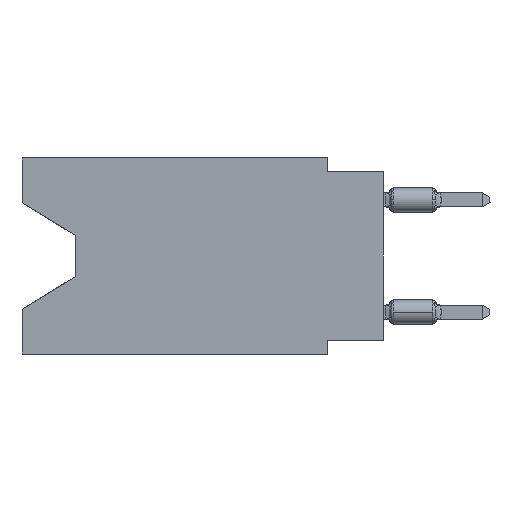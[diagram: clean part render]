
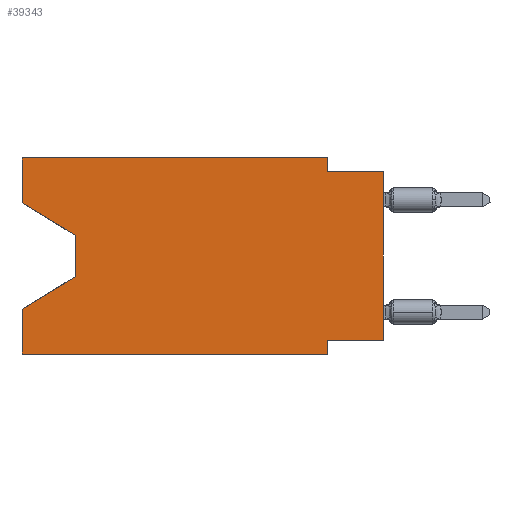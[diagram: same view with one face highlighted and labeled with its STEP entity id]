
A CAD part, left-side view. The second image highlights one B-rep face of the part: STEP entity #39343.
In plain terms, the highlighted planar face has unit normal (-1, 0, 0).
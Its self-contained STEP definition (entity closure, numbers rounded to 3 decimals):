
#518 = DIRECTION ( 'NONE',  ( 0., -1., 0. ) ) ;
#731 = DIRECTION ( 'NONE',  ( 0., -1., 0. ) ) ;
#1422 = CARTESIAN_POINT ( 'NONE',  ( 0., 13.97, -3.505 ) ) ;
#1849 = VERTEX_POINT ( 'NONE', #2627 ) ;
#1996 = VECTOR ( 'NONE', #51085, 1000. ) ;
#2087 = EDGE_LOOP ( 'NONE', ( #16114, #37266, #36667, #16920, #6599, #61075, #36637, #40089, #30793, #2458, #24919, #53079 ) ) ;
#2458 = ORIENTED_EDGE ( 'NONE', *, *, #10654, .F. ) ;
#2627 = CARTESIAN_POINT ( 'NONE',  ( 0., 2.54, -8.255 ) ) ;
#3861 = CARTESIAN_POINT ( 'NONE',  ( 0., 16.383, -8.89 ) ) ;
#4676 = CARTESIAN_POINT ( 'NONE',  ( 0., 0., -0.635 ) ) ;
#5879 = LINE ( 'NONE', #40136, #1996 ) ;
#6353 = CARTESIAN_POINT ( 'NONE',  ( 0., 16.383, -8.89 ) ) ;
#6599 = ORIENTED_EDGE ( 'NONE', *, *, #56846, .T. ) ;
#6923 = CARTESIAN_POINT ( 'NONE',  ( 0., 16.383, 0. ) ) ;
#7086 = LINE ( 'NONE', #69049, #21964 ) ;
#8711 = LINE ( 'NONE', #36781, #38180 ) ;
#8749 = DIRECTION ( 'NONE',  ( 0., 0., -1. ) ) ;
#9603 = CARTESIAN_POINT ( 'NONE',  ( 0., 16.383, -2.038 ) ) ;
#10057 = DIRECTION ( 'NONE',  ( 0., 0., -1. ) ) ;
#10330 = DIRECTION ( 'NONE',  ( 0., 0., 1. ) ) ;
#10654 = EDGE_CURVE ( 'NONE', #14578, #63282, #7086, .T. ) ;
#12421 = VECTOR ( 'NONE', #10057, 1000. ) ;
#12551 = EDGE_CURVE ( 'NONE', #14363, #37885, #18939, .T. ) ;
#12868 = VERTEX_POINT ( 'NONE', #9603 ) ;
#13002 = CARTESIAN_POINT ( 'NONE',  ( 0., 16.383, 0. ) ) ;
#14363 = VERTEX_POINT ( 'NONE', #3861 ) ;
#14437 = VECTOR ( 'NONE', #518, 1000. ) ;
#14578 = VERTEX_POINT ( 'NONE', #28635 ) ;
#14747 = LINE ( 'NONE', #59226, #44307 ) ;
#15629 = VECTOR ( 'NONE', #36415, 1000. ) ;
#16114 = ORIENTED_EDGE ( 'NONE', *, *, #65312, .T. ) ;
#16920 = ORIENTED_EDGE ( 'NONE', *, *, #12551, .F. ) ;
#17519 = LINE ( 'NONE', #56531, #51756 ) ;
#17659 = VECTOR ( 'NONE', #30242, 1000. ) ;
#18939 = LINE ( 'NONE', #57948, #17659 ) ;
#19526 = VERTEX_POINT ( 'NONE', #44234 ) ;
#20314 = CARTESIAN_POINT ( 'NONE',  ( 0., 13.97, -5.385 ) ) ;
#21296 = EDGE_CURVE ( 'NONE', #25168, #22337, #37775, .T. ) ;
#21964 = VECTOR ( 'NONE', #52293, 1000. ) ;
#22337 = VERTEX_POINT ( 'NONE', #20314 ) ;
#24919 = ORIENTED_EDGE ( 'NONE', *, *, #62285, .F. ) ;
#25168 = VERTEX_POINT ( 'NONE', #1422 ) ;
#26548 = EDGE_CURVE ( 'NONE', #22337, #37885, #8711, .T. ) ;
#27928 = CARTESIAN_POINT ( 'NONE',  ( 0., 2.54, -0.635 ) ) ;
#28635 = CARTESIAN_POINT ( 'NONE',  ( 0., 2.54, 0. ) ) ;
#29159 = DIRECTION ( 'NONE',  ( 0., 0., -1. ) ) ;
#29641 = VERTEX_POINT ( 'NONE', #70149 ) ;
#30242 = DIRECTION ( 'NONE',  ( 0., 0., 1. ) ) ;
#30793 = ORIENTED_EDGE ( 'NONE', *, *, #40383, .F. ) ;
#31771 = VECTOR ( 'NONE', #10330, 1000. ) ;
#31847 = CARTESIAN_POINT ( 'NONE',  ( 0., 0., 0. ) ) ;
#35004 = EDGE_CURVE ( 'NONE', #19526, #1849, #5879, .T. ) ;
#35238 = VECTOR ( 'NONE', #47574, 1000. ) ;
#35347 = LINE ( 'NONE', #45940, #15629 ) ;
#36104 = CARTESIAN_POINT ( 'NONE',  ( 0., 2.54, -8.89 ) ) ;
#36415 = DIRECTION ( 'NONE',  ( 0., 0., 1. ) ) ;
#36637 = ORIENTED_EDGE ( 'NONE', *, *, #35004, .F. ) ;
#36667 = ORIENTED_EDGE ( 'NONE', *, *, #26548, .T. ) ;
#36781 = CARTESIAN_POINT ( 'NONE',  ( 0., 13.97, -5.385 ) ) ;
#37266 = ORIENTED_EDGE ( 'NONE', *, *, #21296, .T. ) ;
#37775 = LINE ( 'NONE', #60020, #12421 ) ;
#37885 = VERTEX_POINT ( 'NONE', #42711 ) ;
#38180 = VECTOR ( 'NONE', #47729, 1000. ) ;
#39218 = EDGE_CURVE ( 'NONE', #19526, #62628, #59557, .T. ) ;
#39343 = ADVANCED_FACE ( 'NONE', ( #55182 ), #56879, .F. ) ;
#40089 = ORIENTED_EDGE ( 'NONE', *, *, #39218, .T. ) ;
#40136 = CARTESIAN_POINT ( 'NONE',  ( 0., 0., -8.255 ) ) ;
#40383 = EDGE_CURVE ( 'NONE', #63282, #62628, #14747, .T. ) ;
#42711 = CARTESIAN_POINT ( 'NONE',  ( 0., 16.383, -6.852 ) ) ;
#44234 = CARTESIAN_POINT ( 'NONE',  ( 0., 0., -8.255 ) ) ;
#44307 = VECTOR ( 'NONE', #58488, 1000. ) ;
#45940 = CARTESIAN_POINT ( 'NONE',  ( 0., 16.383, 0. ) ) ;
#46505 = CARTESIAN_POINT ( 'NONE',  ( 0., 16.383, -2.038 ) ) ;
#47228 = LINE ( 'NONE', #46505, #35238 ) ;
#47574 = DIRECTION ( 'NONE',  ( 0., -0.855, -0.519 ) ) ;
#47729 = DIRECTION ( 'NONE',  ( 0., 0.855, -0.519 ) ) ;
#51085 = DIRECTION ( 'NONE',  ( 0., 1., 0. ) ) ;
#51756 = VECTOR ( 'NONE', #731, 1000. ) ;
#52293 = DIRECTION ( 'NONE',  ( 0., 0., -1. ) ) ;
#53079 = ORIENTED_EDGE ( 'NONE', *, *, #62569, .F. ) ;
#54475 = DIRECTION ( 'NONE',  ( 1., 0., 0. ) ) ;
#55182 = FACE_OUTER_BOUND ( 'NONE', #2087, .T. ) ;
#56531 = CARTESIAN_POINT ( 'NONE',  ( 0., 16.383, 0. ) ) ;
#56846 = EDGE_CURVE ( 'NONE', #14363, #29641, #61766, .T. ) ;
#56879 = PLANE ( 'NONE',  #60500 ) ;
#57948 = CARTESIAN_POINT ( 'NONE',  ( 0., 16.383, 0. ) ) ;
#58488 = DIRECTION ( 'NONE',  ( 0., -1., 0. ) ) ;
#59226 = CARTESIAN_POINT ( 'NONE',  ( 0., 0., -0.635 ) ) ;
#59557 = LINE ( 'NONE', #31847, #31771 ) ;
#60020 = CARTESIAN_POINT ( 'NONE',  ( 0., 13.97, -3.505 ) ) ;
#60500 = AXIS2_PLACEMENT_3D ( 'NONE', #6923, #54475, #29159 ) ;
#61075 = ORIENTED_EDGE ( 'NONE', *, *, #70982, .F. ) ;
#61747 = VERTEX_POINT ( 'NONE', #13002 ) ;
#61766 = LINE ( 'NONE', #6353, #14437 ) ;
#62285 = EDGE_CURVE ( 'NONE', #61747, #14578, #17519, .T. ) ;
#62569 = EDGE_CURVE ( 'NONE', #12868, #61747, #35347, .T. ) ;
#62628 = VERTEX_POINT ( 'NONE', #4676 ) ;
#63282 = VERTEX_POINT ( 'NONE', #27928 ) ;
#63807 = LINE ( 'NONE', #36104, #70945 ) ;
#65312 = EDGE_CURVE ( 'NONE', #12868, #25168, #47228, .T. ) ;
#69049 = CARTESIAN_POINT ( 'NONE',  ( 0., 2.54, 0. ) ) ;
#70149 = CARTESIAN_POINT ( 'NONE',  ( 0., 2.54, -8.89 ) ) ;
#70945 = VECTOR ( 'NONE', #8749, 1000. ) ;
#70982 = EDGE_CURVE ( 'NONE', #1849, #29641, #63807, .T. ) ;
